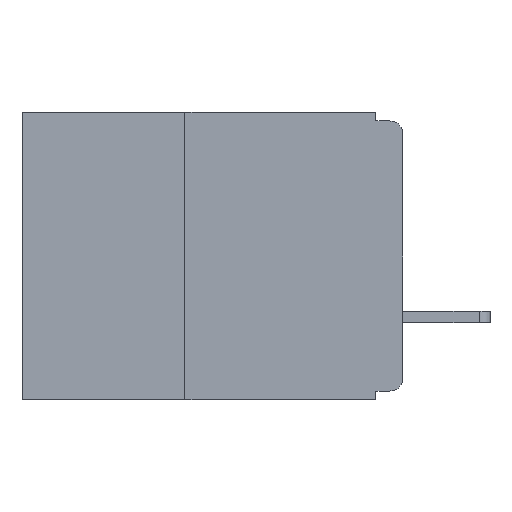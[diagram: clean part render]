
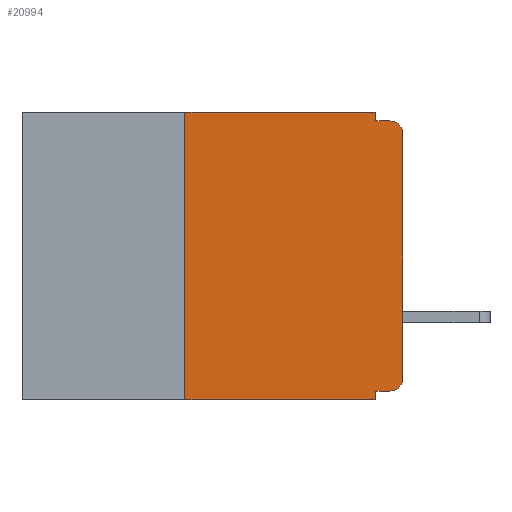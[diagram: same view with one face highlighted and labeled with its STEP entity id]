
A CAD part, left-side view. The second image highlights one B-rep face of the part: STEP entity #20994.
In plain terms, the highlighted planar face has unit normal (-1, 0, 0).
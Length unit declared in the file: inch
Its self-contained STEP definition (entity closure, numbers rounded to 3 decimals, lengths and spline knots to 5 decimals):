
#704 = VERTEX_POINT ( 'NONE', #17348 ) ;
#1095 = ORIENTED_EDGE ( 'NONE', *, *, #2136, .F. ) ;
#1142 = LINE ( 'NONE', #19486, #24080 ) ;
#2013 = ORIENTED_EDGE ( 'NONE', *, *, #14463, .F. ) ;
#2136 = EDGE_CURVE ( 'NONE', #18210, #11887, #1142, .T. ) ;
#2194 = DIRECTION ( 'NONE',  ( 0., 0., 1. ) ) ;
#2287 = CARTESIAN_POINT ( 'NONE',  ( 0., 0., 0. ) ) ;
#2451 = LINE ( 'NONE', #11964, #25406 ) ;
#3334 = AXIS2_PLACEMENT_3D ( 'NONE', #18679, #5264, #20868 ) ;
#3368 = CARTESIAN_POINT ( 'NONE',  ( 0., 0., -0.305 ) ) ;
#3539 = ORIENTED_EDGE ( 'NONE', *, *, #8083, .F. ) ;
#3633 = EDGE_CURVE ( 'NONE', #4831, #11887, #24715, .T. ) ;
#4184 = DIRECTION ( 'NONE',  ( 0., -1., 0. ) ) ;
#4187 = EDGE_CURVE ( 'NONE', #12718, #11353, #14633, .T. ) ;
#4831 = VERTEX_POINT ( 'NONE', #20268 ) ;
#4933 = CARTESIAN_POINT ( 'NONE',  ( 0., 0.031, -0.33 ) ) ;
#5197 = VERTEX_POINT ( 'NONE', #21723 ) ;
#5264 = DIRECTION ( 'NONE',  ( -1., 0., 0. ) ) ;
#6637 = CARTESIAN_POINT ( 'NONE',  ( 0., 0.031, 0. ) ) ;
#6823 = CARTESIAN_POINT ( 'NONE',  ( 0., 0.25, -0.33 ) ) ;
#6936 = VECTOR ( 'NONE', #14719, 39.37008 ) ;
#7761 = VERTEX_POINT ( 'NONE', #14594 ) ;
#8083 = EDGE_CURVE ( 'NONE', #4831, #704, #27464, .T. ) ;
#8143 = DIRECTION ( 'NONE',  ( -1., 0., 0. ) ) ;
#8482 = CARTESIAN_POINT ( 'NONE',  ( 0., 0.031, -0.32 ) ) ;
#8945 = ORIENTED_EDGE ( 'NONE', *, *, #18228, .F. ) ;
#9159 = ORIENTED_EDGE ( 'NONE', *, *, #3633, .T. ) ;
#9368 = VECTOR ( 'NONE', #2194, 39.37008 ) ;
#9690 = ORIENTED_EDGE ( 'NONE', *, *, #11328, .T. ) ;
#9694 = PLANE ( 'NONE',  #22741 ) ;
#10393 = CARTESIAN_POINT ( 'NONE',  ( 0., 0., -0.32 ) ) ;
#11107 = EDGE_CURVE ( 'NONE', #5197, #21578, #25593, .T. ) ;
#11328 = EDGE_CURVE ( 'NONE', #21226, #12718, #18691, .T. ) ;
#11353 = VERTEX_POINT ( 'NONE', #14175 ) ;
#11887 = VERTEX_POINT ( 'NONE', #4933 ) ;
#11964 = CARTESIAN_POINT ( 'NONE',  ( 0., 0.437, 0. ) ) ;
#11978 = DIRECTION ( 'NONE',  ( 1., 0., 0. ) ) ;
#12545 = VECTOR ( 'NONE', #4184, 39.37008 ) ;
#12716 = FACE_OUTER_BOUND ( 'NONE', #14860, .T. ) ;
#12718 = VERTEX_POINT ( 'NONE', #3368 ) ;
#13121 = VECTOR ( 'NONE', #24466, 39.37008 ) ;
#13504 = DIRECTION ( 'NONE',  ( 0., 0., 1. ) ) ;
#14175 = CARTESIAN_POINT ( 'NONE',  ( 0., 0., -0.025 ) ) ;
#14463 = EDGE_CURVE ( 'NONE', #704, #5197, #2451, .T. ) ;
#14594 = CARTESIAN_POINT ( 'NONE',  ( 0., 0.015, -0.01 ) ) ;
#14633 = LINE ( 'NONE', #2287, #9368 ) ;
#14719 = DIRECTION ( 'NONE',  ( 0., -1., 0. ) ) ;
#14860 = EDGE_LOOP ( 'NONE', ( #24747, #21322, #8945, #28024, #2013, #3539, #9159, #1095, #21132, #9690 ) ) ;
#15100 = CARTESIAN_POINT ( 'NONE',  ( 0., 0.437, -0.33 ) ) ;
#15605 = CIRCLE ( 'NONE', #23789, 0.015 ) ;
#17348 = CARTESIAN_POINT ( 'NONE',  ( 0., 0.25, 0. ) ) ;
#17600 = VECTOR ( 'NONE', #28037, 39.37008 ) ;
#18210 = VERTEX_POINT ( 'NONE', #8482 ) ;
#18228 = EDGE_CURVE ( 'NONE', #21578, #7761, #18454, .T. ) ;
#18315 = CARTESIAN_POINT ( 'NONE',  ( 0., 0.031, -0.01 ) ) ;
#18454 = LINE ( 'NONE', #28545, #12545 ) ;
#18679 = CARTESIAN_POINT ( 'NONE',  ( 0., 0.015, -0.305 ) ) ;
#18691 = CIRCLE ( 'NONE', #3334, 0.015 ) ;
#18803 = EDGE_CURVE ( 'NONE', #11353, #7761, #15605, .T. ) ;
#19479 = DIRECTION ( 'NONE',  ( 0., 0., -1. ) ) ;
#19486 = CARTESIAN_POINT ( 'NONE',  ( 0., 0.031, -0.33 ) ) ;
#20268 = CARTESIAN_POINT ( 'NONE',  ( 0., 0.25, -0.33 ) ) ;
#20868 = DIRECTION ( 'NONE',  ( 0., 0., -1. ) ) ;
#20885 = DIRECTION ( 'NONE',  ( 0., -1., 0. ) ) ;
#20994 = ADVANCED_FACE ( 'NONE', ( #12716 ), #9694, .F. ) ;
#21132 = ORIENTED_EDGE ( 'NONE', *, *, #26169, .F. ) ;
#21226 = VERTEX_POINT ( 'NONE', #25999 ) ;
#21322 = ORIENTED_EDGE ( 'NONE', *, *, #18803, .T. ) ;
#21507 = CARTESIAN_POINT ( 'NONE',  ( 0., 0.015, -0.025 ) ) ;
#21578 = VERTEX_POINT ( 'NONE', #18315 ) ;
#21723 = CARTESIAN_POINT ( 'NONE',  ( 0., 0.031, 0. ) ) ;
#22741 = AXIS2_PLACEMENT_3D ( 'NONE', #25247, #11978, #27422 ) ;
#23720 = DIRECTION ( 'NONE',  ( 0., 0., -1. ) ) ;
#23789 = AXIS2_PLACEMENT_3D ( 'NONE', #21507, #8143, #23720 ) ;
#24080 = VECTOR ( 'NONE', #19479, 39.37008 ) ;
#24466 = DIRECTION ( 'NONE',  ( 0., 0., -1. ) ) ;
#24715 = LINE ( 'NONE', #15100, #6936 ) ;
#24747 = ORIENTED_EDGE ( 'NONE', *, *, #4187, .T. ) ;
#24861 = LINE ( 'NONE', #10393, #17600 ) ;
#25247 = CARTESIAN_POINT ( 'NONE',  ( 0., 0.437, 0. ) ) ;
#25406 = VECTOR ( 'NONE', #20885, 39.37008 ) ;
#25593 = LINE ( 'NONE', #6637, #13121 ) ;
#25999 = CARTESIAN_POINT ( 'NONE',  ( 0., 0.015, -0.32 ) ) ;
#26169 = EDGE_CURVE ( 'NONE', #21226, #18210, #24861, .T. ) ;
#26779 = VECTOR ( 'NONE', #13504, 39.37008 ) ;
#27422 = DIRECTION ( 'NONE',  ( 0., 0., -1. ) ) ;
#27464 = LINE ( 'NONE', #6823, #26779 ) ;
#28024 = ORIENTED_EDGE ( 'NONE', *, *, #11107, .F. ) ;
#28037 = DIRECTION ( 'NONE',  ( 0., 1., 0. ) ) ;
#28545 = CARTESIAN_POINT ( 'NONE',  ( 0., 0., -0.01 ) ) ;
